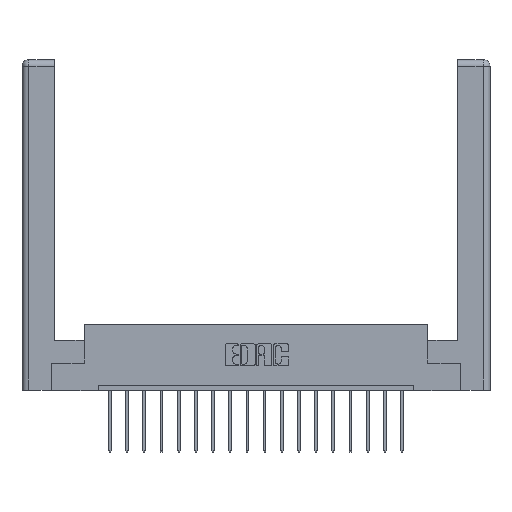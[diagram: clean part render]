
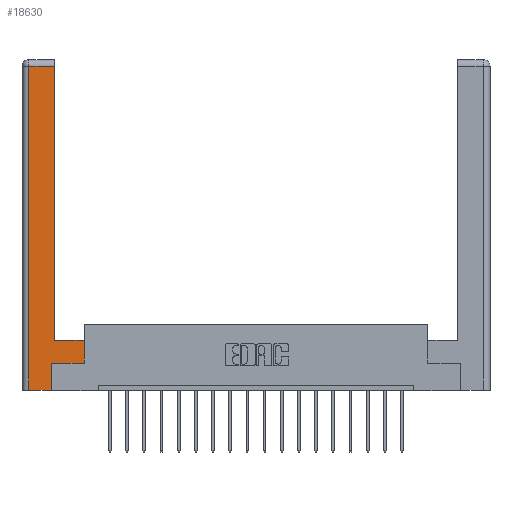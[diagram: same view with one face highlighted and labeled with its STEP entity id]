
A CAD part, top view. The second image highlights one B-rep face of the part: STEP entity #18630.
In plain terms, the highlighted planar face has unit normal (0, 0, 1).
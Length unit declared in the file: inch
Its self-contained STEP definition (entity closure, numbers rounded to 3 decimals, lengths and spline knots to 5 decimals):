
#236 = ORIENTED_EDGE ( 'NONE', *, *, #3631, .T. ) ;
#696 = CARTESIAN_POINT ( 'NONE',  ( 0.0615, 2.94, 0. ) ) ;
#1064 = ORIENTED_EDGE ( 'NONE', *, *, #15656, .T. ) ;
#1551 = CARTESIAN_POINT ( 'NONE',  ( 0.565, 0.245, 0. ) ) ;
#1593 = EDGE_CURVE ( 'NONE', #13751, #13285, #9285, .T. ) ;
#1808 = VECTOR ( 'NONE', #3781, 39.37008 ) ;
#2098 = VERTEX_POINT ( 'NONE', #11207 ) ;
#2846 = VERTEX_POINT ( 'NONE', #9874 ) ;
#3478 = CARTESIAN_POINT ( 'NONE',  ( 0., 0., 0. ) ) ;
#3631 = EDGE_CURVE ( 'NONE', #4021, #12618, #10829, .T. ) ;
#3781 = DIRECTION ( 'NONE',  ( 1., 0., 0. ) ) ;
#3807 = CARTESIAN_POINT ( 'NONE',  ( 0.295, 0.45, 0. ) ) ;
#4021 = VERTEX_POINT ( 'NONE', #18934 ) ;
#4506 = EDGE_CURVE ( 'NONE', #18507, #2846, #5832, .T. ) ;
#4733 = LINE ( 'NONE', #16151, #5671 ) ;
#4953 = DIRECTION ( 'NONE',  ( 0., 1., 0. ) ) ;
#5138 = CARTESIAN_POINT ( 'NONE',  ( 0.265, 0., 0. ) ) ;
#5231 = LINE ( 'NONE', #6375, #18652 ) ;
#5671 = VECTOR ( 'NONE', #10235, 39.37008 ) ;
#5832 = LINE ( 'NONE', #6616, #13517 ) ;
#6375 = CARTESIAN_POINT ( 'NONE',  ( 0.265, 0.245, 0. ) ) ;
#6509 = EDGE_CURVE ( 'NONE', #2098, #13751, #15498, .T. ) ;
#6616 = CARTESIAN_POINT ( 'NONE',  ( 0.0615, 0., 0. ) ) ;
#7581 = VERTEX_POINT ( 'NONE', #5138 ) ;
#7591 = EDGE_CURVE ( 'NONE', #2846, #7581, #12885, .T. ) ;
#7771 = EDGE_CURVE ( 'NONE', #13285, #4021, #16376, .T. ) ;
#7875 = DIRECTION ( 'NONE',  ( 0., 1., 0. ) ) ;
#7969 = EDGE_LOOP ( 'NONE', ( #236, #12841, #11147, #14794, #1064, #17178, #16590, #15583 ) ) ;
#8130 = CARTESIAN_POINT ( 'NONE',  ( 0.565, 0.45, 0. ) ) ;
#8216 = EDGE_CURVE ( 'NONE', #12618, #18507, #4733, .T. ) ;
#8713 = VECTOR ( 'NONE', #18401, 39.37008 ) ;
#9285 = LINE ( 'NONE', #8130, #14894 ) ;
#9753 = CARTESIAN_POINT ( 'NONE',  ( 0.265, 0., 0. ) ) ;
#9874 = CARTESIAN_POINT ( 'NONE',  ( 0.0615, 0., 0. ) ) ;
#10235 = DIRECTION ( 'NONE',  ( -1., 0., 0. ) ) ;
#10378 = VECTOR ( 'NONE', #12636, 39.37008 ) ;
#10776 = CARTESIAN_POINT ( 'NONE',  ( 0.565, 0.45, 0. ) ) ;
#10792 = FACE_OUTER_BOUND ( 'NONE', #7969, .T. ) ;
#10829 = LINE ( 'NONE', #11142, #10378 ) ;
#10902 = DIRECTION ( 'NONE',  ( 0., -1., 0. ) ) ;
#11142 = CARTESIAN_POINT ( 'NONE',  ( 0.295, 3., 0. ) ) ;
#11147 = ORIENTED_EDGE ( 'NONE', *, *, #4506, .T. ) ;
#11207 = CARTESIAN_POINT ( 'NONE',  ( 0.265, 0.245, 0. ) ) ;
#11374 = DIRECTION ( 'NONE',  ( 0., 0., -1. ) ) ;
#12415 = PLANE ( 'NONE',  #16247 ) ;
#12618 = VERTEX_POINT ( 'NONE', #12622 ) ;
#12622 = CARTESIAN_POINT ( 'NONE',  ( 0.295, 2.94, 0. ) ) ;
#12636 = DIRECTION ( 'NONE',  ( 0., 1., 0. ) ) ;
#12841 = ORIENTED_EDGE ( 'NONE', *, *, #8216, .T. ) ;
#12885 = LINE ( 'NONE', #9753, #8713 ) ;
#13285 = VERTEX_POINT ( 'NONE', #10776 ) ;
#13517 = VECTOR ( 'NONE', #10902, 39.37008 ) ;
#13751 = VERTEX_POINT ( 'NONE', #1551 ) ;
#14033 = CARTESIAN_POINT ( 'NONE',  ( 0.565, 0.245, 0. ) ) ;
#14295 = VECTOR ( 'NONE', #15525, 39.37008 ) ;
#14794 = ORIENTED_EDGE ( 'NONE', *, *, #7591, .T. ) ;
#14894 = VECTOR ( 'NONE', #4953, 39.37008 ) ;
#15498 = LINE ( 'NONE', #14033, #1808 ) ;
#15525 = DIRECTION ( 'NONE',  ( -1., 0., 0. ) ) ;
#15583 = ORIENTED_EDGE ( 'NONE', *, *, #7771, .T. ) ;
#15656 = EDGE_CURVE ( 'NONE', #7581, #2098, #5231, .T. ) ;
#16151 = CARTESIAN_POINT ( 'NONE',  ( 0.0615, 2.94, 0. ) ) ;
#16247 = AXIS2_PLACEMENT_3D ( 'NONE', #3478, #11374, #17190 ) ;
#16376 = LINE ( 'NONE', #3807, #14295 ) ;
#16590 = ORIENTED_EDGE ( 'NONE', *, *, #1593, .T. ) ;
#17178 = ORIENTED_EDGE ( 'NONE', *, *, #6509, .T. ) ;
#17190 = DIRECTION ( 'NONE',  ( -1., 0., 0. ) ) ;
#18401 = DIRECTION ( 'NONE',  ( 1., 0., 0. ) ) ;
#18507 = VERTEX_POINT ( 'NONE', #696 ) ;
#18630 = ADVANCED_FACE ( 'NONE', ( #10792 ), #12415, .F. ) ;
#18652 = VECTOR ( 'NONE', #7875, 39.37008 ) ;
#18934 = CARTESIAN_POINT ( 'NONE',  ( 0.295, 0.45, 0. ) ) ;
